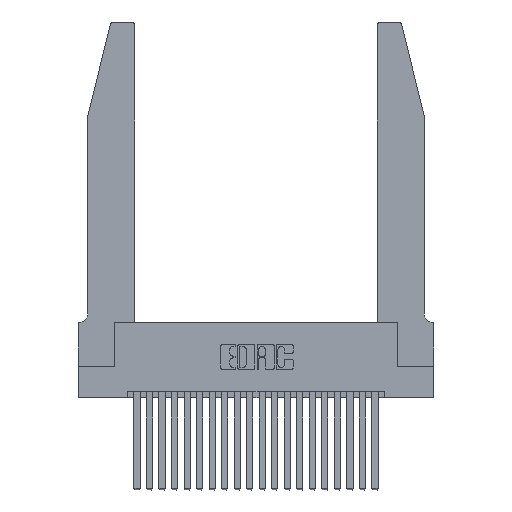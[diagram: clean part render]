
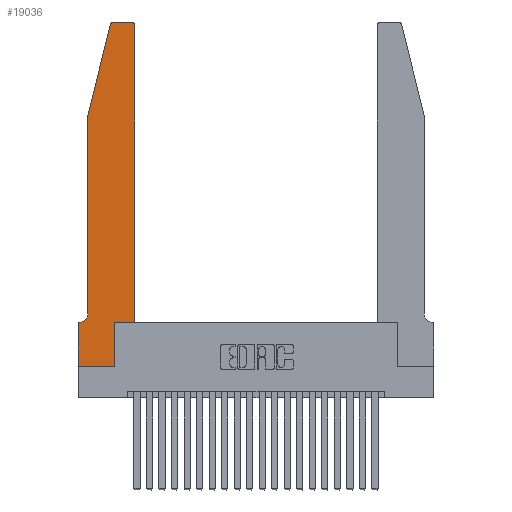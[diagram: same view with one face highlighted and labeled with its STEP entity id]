
A CAD part, top view. The second image highlights one B-rep face of the part: STEP entity #19036.
In plain terms, the highlighted planar face has unit normal (0, 0, 1).
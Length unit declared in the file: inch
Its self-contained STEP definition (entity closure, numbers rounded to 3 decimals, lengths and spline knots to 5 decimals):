
#85 = CARTESIAN_POINT ( 'NONE',  ( 0.0755, 2., 0.37 ) ) ;
#144 = EDGE_CURVE ( 'NONE', #2782, #19047, #385, .T. ) ;
#385 = CIRCLE ( 'NONE', #2526, 0.03 ) ;
#652 = CARTESIAN_POINT ( 'NONE',  ( 0.25487, 2.72718, 0.37 ) ) ;
#985 = CIRCLE ( 'NONE', #13314, 0.07 ) ;
#1454 = LINE ( 'NONE', #85, #14927 ) ;
#1515 = CARTESIAN_POINT ( 'NONE',  ( 0.0755, 0.35, 0.37 ) ) ;
#1741 = CARTESIAN_POINT ( 'NONE',  ( 0., 0.35, 0.37 ) ) ;
#1955 = LINE ( 'NONE', #12145, #11795 ) ;
#2022 = EDGE_CURVE ( 'NONE', #21080, #2186, #1955, .T. ) ;
#2099 = ORIENTED_EDGE ( 'NONE', *, *, #13498, .T. ) ;
#2186 = VERTEX_POINT ( 'NONE', #13510 ) ;
#2408 = LINE ( 'NONE', #17875, #16340 ) ;
#2526 = AXIS2_PLACEMENT_3D ( 'NONE', #20076, #2972, #12157 ) ;
#2655 = CARTESIAN_POINT ( 'NONE',  ( 0.0755, 0.42, 0.37 ) ) ;
#2781 = VECTOR ( 'NONE', #20704, 39.37008 ) ;
#2782 = VERTEX_POINT ( 'NONE', #3291 ) ;
#2944 = ORIENTED_EDGE ( 'NONE', *, *, #4213, .T. ) ;
#2972 = DIRECTION ( 'NONE',  ( 0., 0., 1. ) ) ;
#2984 = DIRECTION ( 'NONE',  ( 0., 0., -1. ) ) ;
#3063 = LINE ( 'NONE', #7067, #21538 ) ;
#3269 = CARTESIAN_POINT ( 'NONE',  ( 0.284, 2.72, 0.37 ) ) ;
#3291 = CARTESIAN_POINT ( 'NONE',  ( 0.4505, 2.72, 0.37 ) ) ;
#3365 = CARTESIAN_POINT ( 'NONE',  ( 0.0755, 2., 0.37 ) ) ;
#3438 = VECTOR ( 'NONE', #22948, 39.37008 ) ;
#4213 = EDGE_CURVE ( 'NONE', #9024, #21160, #3063, .T. ) ;
#4540 = ORIENTED_EDGE ( 'NONE', *, *, #144, .T. ) ;
#4663 = VECTOR ( 'NONE', #18407, 39.37008 ) ;
#5144 = DIRECTION ( 'NONE',  ( 1., 0., 0. ) ) ;
#5916 = ORIENTED_EDGE ( 'NONE', *, *, #11154, .T. ) ;
#6431 = ORIENTED_EDGE ( 'NONE', *, *, #7625, .T. ) ;
#6628 = VERTEX_POINT ( 'NONE', #6630 ) ;
#6630 = CARTESIAN_POINT ( 'NONE',  ( 0.0055, 0.35, 0.37 ) ) ;
#6838 = ORIENTED_EDGE ( 'NONE', *, *, #7294, .T. ) ;
#7067 = CARTESIAN_POINT ( 'NONE',  ( 0.0755, 2., 0.37 ) ) ;
#7294 = EDGE_CURVE ( 'NONE', #13049, #9024, #10442, .T. ) ;
#7625 = EDGE_CURVE ( 'NONE', #2186, #8998, #14921, .T. ) ;
#7710 = CARTESIAN_POINT ( 'NONE',  ( 0.2605, 2.75, 0.37 ) ) ;
#7728 = CARTESIAN_POINT ( 'NONE',  ( 0.2865, 0.35, 0.37 ) ) ;
#8258 = DIRECTION ( 'NONE',  ( 0., 0., 1. ) ) ;
#8742 = VERTEX_POINT ( 'NONE', #1741 ) ;
#8998 = VERTEX_POINT ( 'NONE', #15160 ) ;
#9024 = VERTEX_POINT ( 'NONE', #652 ) ;
#9881 = CARTESIAN_POINT ( 'NONE',  ( 0.284, 2.75, 0.37 ) ) ;
#10103 = DIRECTION ( 'NONE',  ( 1., 0., 0. ) ) ;
#10195 = CARTESIAN_POINT ( 'NONE',  ( 0.4505, 0.35, 0.37 ) ) ;
#10442 = CIRCLE ( 'NONE', #20381, 0.03 ) ;
#10472 = CARTESIAN_POINT ( 'NONE',  ( 0., 0., 0.37 ) ) ;
#10503 = CARTESIAN_POINT ( 'NONE',  ( 0.4505, 0.35, 0.37 ) ) ;
#10639 = ORIENTED_EDGE ( 'NONE', *, *, #20024, .T. ) ;
#11154 = EDGE_CURVE ( 'NONE', #22182, #6628, #985, .T. ) ;
#11795 = VECTOR ( 'NONE', #10103, 39.37008 ) ;
#11833 = LINE ( 'NONE', #7710, #20565 ) ;
#11931 = CARTESIAN_POINT ( 'NONE',  ( 0.4205, 2.75, 0.37 ) ) ;
#12145 = CARTESIAN_POINT ( 'NONE',  ( 0., 0., 0.37 ) ) ;
#12157 = DIRECTION ( 'NONE',  ( 1., 0., 0. ) ) ;
#12358 = DIRECTION ( 'NONE',  ( 1., 0., 0. ) ) ;
#12579 = ORIENTED_EDGE ( 'NONE', *, *, #2022, .T. ) ;
#13040 = DIRECTION ( 'NONE',  ( 0., -1., 0. ) ) ;
#13049 = VERTEX_POINT ( 'NONE', #9881 ) ;
#13282 = EDGE_CURVE ( 'NONE', #8998, #18885, #19260, .T. ) ;
#13314 = AXIS2_PLACEMENT_3D ( 'NONE', #13969, #2984, #15719 ) ;
#13498 = EDGE_CURVE ( 'NONE', #21160, #22182, #1454, .T. ) ;
#13510 = CARTESIAN_POINT ( 'NONE',  ( 0.2865, 0., 0.37 ) ) ;
#13742 = FACE_OUTER_BOUND ( 'NONE', #18563, .T. ) ;
#13969 = CARTESIAN_POINT ( 'NONE',  ( 0.0055, 0.42, 0.37 ) ) ;
#14523 = ORIENTED_EDGE ( 'NONE', *, *, #16071, .T. ) ;
#14662 = VECTOR ( 'NONE', #12358, 39.37008 ) ;
#14902 = DIRECTION ( 'NONE',  ( -1., 0., 0. ) ) ;
#14921 = LINE ( 'NONE', #7728, #4663 ) ;
#14927 = VECTOR ( 'NONE', #13040, 39.37008 ) ;
#14943 = ORIENTED_EDGE ( 'NONE', *, *, #21982, .T. ) ;
#15011 = EDGE_CURVE ( 'NONE', #6628, #8742, #17843, .T. ) ;
#15160 = CARTESIAN_POINT ( 'NONE',  ( 0.2865, 0.35, 0.37 ) ) ;
#15719 = DIRECTION ( 'NONE',  ( -1., 0., 0. ) ) ;
#15978 = DIRECTION ( 'NONE',  ( 0., 0., 1. ) ) ;
#16071 = EDGE_CURVE ( 'NONE', #8742, #21080, #2408, .T. ) ;
#16340 = VECTOR ( 'NONE', #23039, 39.37008 ) ;
#17843 = LINE ( 'NONE', #1515, #3438 ) ;
#17875 = CARTESIAN_POINT ( 'NONE',  ( 0., 0., 0.37 ) ) ;
#18407 = DIRECTION ( 'NONE',  ( 0., 1., 0. ) ) ;
#18433 = ORIENTED_EDGE ( 'NONE', *, *, #13282, .T. ) ;
#18563 = EDGE_LOOP ( 'NONE', ( #14943, #6838, #2944, #2099, #5916, #21064, #14523, #12579, #6431, #18433, #10639, #4540 ) ) ;
#18885 = VERTEX_POINT ( 'NONE', #21671 ) ;
#18898 = CARTESIAN_POINT ( 'NONE',  ( 0., 0.35, 0.37 ) ) ;
#19036 = ADVANCED_FACE ( 'NONE', ( #13742 ), #20548, .T. ) ;
#19047 = VERTEX_POINT ( 'NONE', #11931 ) ;
#19260 = LINE ( 'NONE', #10503, #14662 ) ;
#19836 = AXIS2_PLACEMENT_3D ( 'NONE', #18898, #8258, #20616 ) ;
#20024 = EDGE_CURVE ( 'NONE', #18885, #2782, #21816, .T. ) ;
#20076 = CARTESIAN_POINT ( 'NONE',  ( 0.4205, 2.72, 0.37 ) ) ;
#20381 = AXIS2_PLACEMENT_3D ( 'NONE', #3269, #15978, #5144 ) ;
#20548 = PLANE ( 'NONE',  #19836 ) ;
#20565 = VECTOR ( 'NONE', #14902, 39.37008 ) ;
#20616 = DIRECTION ( 'NONE',  ( 1., 0., 0. ) ) ;
#20704 = DIRECTION ( 'NONE',  ( 0., 1., 0. ) ) ;
#21064 = ORIENTED_EDGE ( 'NONE', *, *, #15011, .T. ) ;
#21080 = VERTEX_POINT ( 'NONE', #10472 ) ;
#21160 = VERTEX_POINT ( 'NONE', #3365 ) ;
#21538 = VECTOR ( 'NONE', #22964, 39.37008 ) ;
#21671 = CARTESIAN_POINT ( 'NONE',  ( 0.4505, 0.35, 0.37 ) ) ;
#21816 = LINE ( 'NONE', #10195, #2781 ) ;
#21982 = EDGE_CURVE ( 'NONE', #19047, #13049, #11833, .T. ) ;
#22182 = VERTEX_POINT ( 'NONE', #2655 ) ;
#22948 = DIRECTION ( 'NONE',  ( -1., 0., 0. ) ) ;
#22964 = DIRECTION ( 'NONE',  ( -0.239, -0.971, 0. ) ) ;
#23039 = DIRECTION ( 'NONE',  ( 0., -1., 0. ) ) ;
